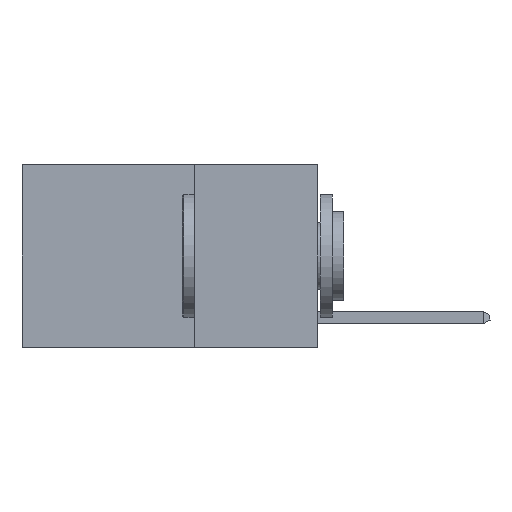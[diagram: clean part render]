
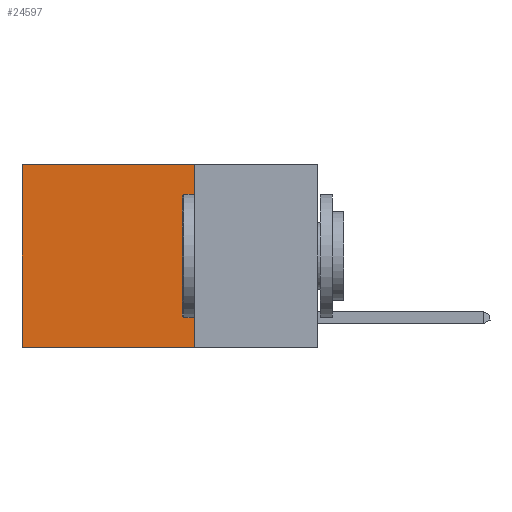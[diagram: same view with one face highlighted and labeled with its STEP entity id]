
A CAD part, left-side view. The second image highlights one B-rep face of the part: STEP entity #24597.
In plain terms, the highlighted planar face has unit normal (-1, 0, 0).
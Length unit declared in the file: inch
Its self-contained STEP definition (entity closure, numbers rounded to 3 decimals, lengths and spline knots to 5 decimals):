
#999 = CARTESIAN_POINT ( 'NONE',  ( 0.2625, 0.25, 0. ) ) ;
#1589 = ORIENTED_EDGE ( 'NONE', *, *, #3276, .T. ) ;
#1653 = FACE_OUTER_BOUND ( 'NONE', #13804, .T. ) ;
#1854 = DIRECTION ( 'NONE',  ( 0., 0., -1. ) ) ;
#1983 = CARTESIAN_POINT ( 'NONE',  ( 0.2625, 0.6, -0.37 ) ) ;
#2457 = LINE ( 'NONE', #7806, #13177 ) ;
#2558 = VERTEX_POINT ( 'NONE', #14595 ) ;
#3241 = CARTESIAN_POINT ( 'NONE',  ( 0.2625, 0.25, -0.37 ) ) ;
#3276 = EDGE_CURVE ( 'NONE', #11587, #11092, #3593, .T. ) ;
#3593 = LINE ( 'NONE', #26237, #20015 ) ;
#6459 = CARTESIAN_POINT ( 'NONE',  ( 0.2625, 0.25, -0.37 ) ) ;
#7464 = DIRECTION ( 'NONE',  ( 0., 0., -1. ) ) ;
#7806 = CARTESIAN_POINT ( 'NONE',  ( 0.2625, 0.25, 0. ) ) ;
#9905 = VERTEX_POINT ( 'NONE', #6459 ) ;
#9964 = VECTOR ( 'NONE', #7464, 39.37008 ) ;
#10642 = LINE ( 'NONE', #999, #9964 ) ;
#10783 = EDGE_CURVE ( 'NONE', #9905, #11092, #12843, .T. ) ;
#10909 = EDGE_CURVE ( 'NONE', #2558, #11587, #2457, .T. ) ;
#11092 = VERTEX_POINT ( 'NONE', #1983 ) ;
#11587 = VERTEX_POINT ( 'NONE', #18541 ) ;
#12843 = LINE ( 'NONE', #3241, #16532 ) ;
#13177 = VECTOR ( 'NONE', #14273, 39.37008 ) ;
#13804 = EDGE_LOOP ( 'NONE', ( #1589, #22908, #19375, #19897 ) ) ;
#13923 = DIRECTION ( 'NONE',  ( 0., 1., 0. ) ) ;
#14273 = DIRECTION ( 'NONE',  ( 0., 1., 0. ) ) ;
#14595 = CARTESIAN_POINT ( 'NONE',  ( 0.2625, 0.25, 0. ) ) ;
#14682 = DIRECTION ( 'NONE',  ( 1., 0., 0. ) ) ;
#16532 = VECTOR ( 'NONE', #13923, 39.37008 ) ;
#16700 = AXIS2_PLACEMENT_3D ( 'NONE', #27479, #14682, #1854 ) ;
#18541 = CARTESIAN_POINT ( 'NONE',  ( 0.2625, 0.6, 0. ) ) ;
#19375 = ORIENTED_EDGE ( 'NONE', *, *, #27709, .F. ) ;
#19897 = ORIENTED_EDGE ( 'NONE', *, *, #10909, .T. ) ;
#20015 = VECTOR ( 'NONE', #21849, 39.37008 ) ;
#21021 = PLANE ( 'NONE',  #16700 ) ;
#21849 = DIRECTION ( 'NONE',  ( 0., 0., -1. ) ) ;
#22908 = ORIENTED_EDGE ( 'NONE', *, *, #10783, .F. ) ;
#24597 = ADVANCED_FACE ( 'NONE', ( #1653 ), #21021, .F. ) ;
#26237 = CARTESIAN_POINT ( 'NONE',  ( 0.2625, 0.6, 0. ) ) ;
#27479 = CARTESIAN_POINT ( 'NONE',  ( 0.2625, 0.25, 0. ) ) ;
#27709 = EDGE_CURVE ( 'NONE', #2558, #9905, #10642, .T. ) ;
